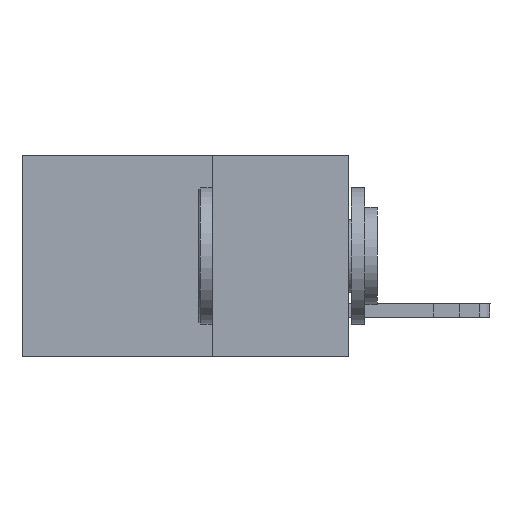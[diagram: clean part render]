
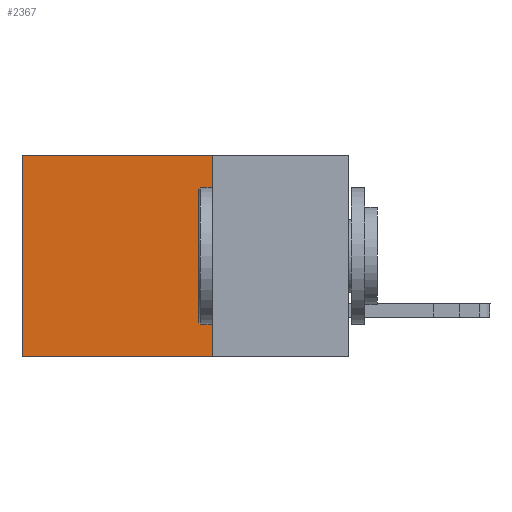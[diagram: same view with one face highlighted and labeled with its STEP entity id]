
A CAD part, left-side view. The second image highlights one B-rep face of the part: STEP entity #2367.
In plain terms, the highlighted planar face has unit normal (-1, 0, 0).
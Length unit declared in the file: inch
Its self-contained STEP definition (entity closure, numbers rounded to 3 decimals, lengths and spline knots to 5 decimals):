
#786 = ORIENTED_EDGE ( 'NONE', *, *, #11255, .F. ) ;
#1557 = LINE ( 'NONE', #10709, #14321 ) ;
#2367 = ADVANCED_FACE ( 'NONE', ( #18314 ), #17129, .F. ) ;
#3114 = VERTEX_POINT ( 'NONE', #16886 ) ;
#3196 = EDGE_CURVE ( 'NONE', #11899, #15469, #9536, .T. ) ;
#3426 = AXIS2_PLACEMENT_3D ( 'NONE', #3500, #7807, #6335 ) ;
#3500 = CARTESIAN_POINT ( 'NONE',  ( 0.298, 0.25, 0. ) ) ;
#4446 = LINE ( 'NONE', #10439, #14437 ) ;
#6260 = EDGE_CURVE ( 'NONE', #15469, #3114, #4446, .T. ) ;
#6335 = DIRECTION ( 'NONE',  ( 0., 0., -1. ) ) ;
#6818 = EDGE_CURVE ( 'NONE', #8392, #3114, #1557, .T. ) ;
#7481 = DIRECTION ( 'NONE',  ( 0., 0., -1. ) ) ;
#7797 = LINE ( 'NONE', #13561, #13184 ) ;
#7807 = DIRECTION ( 'NONE',  ( 1., 0., 0. ) ) ;
#8392 = VERTEX_POINT ( 'NONE', #14676 ) ;
#8723 = VECTOR ( 'NONE', #15293, 39.37008 ) ;
#9536 = LINE ( 'NONE', #10928, #8723 ) ;
#10439 = CARTESIAN_POINT ( 'NONE',  ( 0.298, 0.6, 0. ) ) ;
#10611 = DIRECTION ( 'NONE',  ( 0., 1., 0. ) ) ;
#10709 = CARTESIAN_POINT ( 'NONE',  ( 0.298, 0.25, -0.37 ) ) ;
#10928 = CARTESIAN_POINT ( 'NONE',  ( 0.298, 0.25, 0. ) ) ;
#11162 = CARTESIAN_POINT ( 'NONE',  ( 0.298, 0.6, 0. ) ) ;
#11255 = EDGE_CURVE ( 'NONE', #11899, #8392, #7797, .T. ) ;
#11899 = VERTEX_POINT ( 'NONE', #19240 ) ;
#13184 = VECTOR ( 'NONE', #18110, 39.37008 ) ;
#13396 = ORIENTED_EDGE ( 'NONE', *, *, #6818, .F. ) ;
#13561 = CARTESIAN_POINT ( 'NONE',  ( 0.298, 0.25, 0. ) ) ;
#14321 = VECTOR ( 'NONE', #10611, 39.37008 ) ;
#14437 = VECTOR ( 'NONE', #7481, 39.37008 ) ;
#14676 = CARTESIAN_POINT ( 'NONE',  ( 0.298, 0.25, -0.37 ) ) ;
#15293 = DIRECTION ( 'NONE',  ( 0., 1., 0. ) ) ;
#15308 = EDGE_LOOP ( 'NONE', ( #16373, #13396, #786, #16443 ) ) ;
#15469 = VERTEX_POINT ( 'NONE', #11162 ) ;
#16373 = ORIENTED_EDGE ( 'NONE', *, *, #6260, .T. ) ;
#16443 = ORIENTED_EDGE ( 'NONE', *, *, #3196, .T. ) ;
#16886 = CARTESIAN_POINT ( 'NONE',  ( 0.298, 0.6, -0.37 ) ) ;
#17129 = PLANE ( 'NONE',  #3426 ) ;
#18110 = DIRECTION ( 'NONE',  ( 0., 0., -1. ) ) ;
#18314 = FACE_OUTER_BOUND ( 'NONE', #15308, .T. ) ;
#19240 = CARTESIAN_POINT ( 'NONE',  ( 0.298, 0.25, 0. ) ) ;
